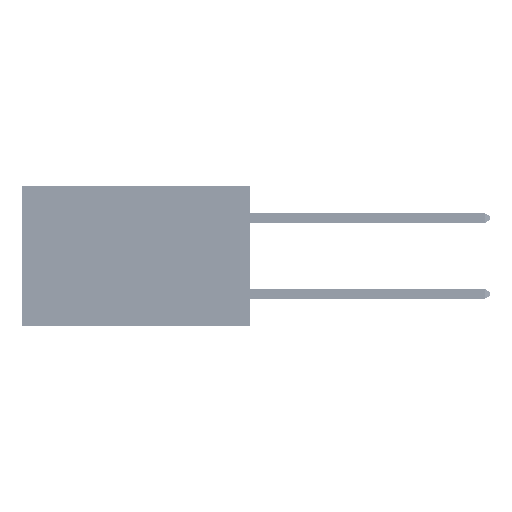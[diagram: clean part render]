
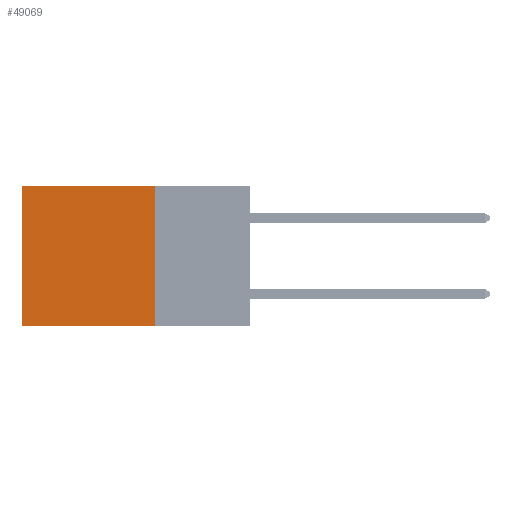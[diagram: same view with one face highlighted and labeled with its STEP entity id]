
A CAD part, left-side view. The second image highlights one B-rep face of the part: STEP entity #49069.
In plain terms, the highlighted planar face has unit normal (-1, 0, 0).
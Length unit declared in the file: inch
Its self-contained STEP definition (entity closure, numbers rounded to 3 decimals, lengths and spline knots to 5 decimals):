
#2378 = CARTESIAN_POINT ( 'NONE',  ( 0.2875, 0.6, 0. ) ) ;
#2854 = DIRECTION ( 'NONE',  ( 0., 1., 0. ) ) ;
#3376 = DIRECTION ( 'NONE',  ( 0., 0., -1. ) ) ;
#6018 = EDGE_LOOP ( 'NONE', ( #32790, #34989, #29587, #33026 ) ) ;
#6453 = LINE ( 'NONE', #21097, #10620 ) ;
#6478 = DIRECTION ( 'NONE',  ( 0., 0., -1. ) ) ;
#7643 = CARTESIAN_POINT ( 'NONE',  ( 0.2875, 0.25, 0. ) ) ;
#9830 = EDGE_CURVE ( 'NONE', #39778, #13255, #45789, .T. ) ;
#9989 = PLANE ( 'NONE',  #31469 ) ;
#10384 = VECTOR ( 'NONE', #3376, 39.37008 ) ;
#10620 = VECTOR ( 'NONE', #32876, 39.37008 ) ;
#13190 = VECTOR ( 'NONE', #18886, 39.37008 ) ;
#13255 = VERTEX_POINT ( 'NONE', #37118 ) ;
#15444 = EDGE_CURVE ( 'NONE', #17338, #19901, #24417, .T. ) ;
#17338 = VERTEX_POINT ( 'NONE', #34936 ) ;
#18886 = DIRECTION ( 'NONE',  ( 0., 1., 0. ) ) ;
#19901 = VERTEX_POINT ( 'NONE', #41632 ) ;
#21097 = CARTESIAN_POINT ( 'NONE',  ( 0.2875, 0.25, 0. ) ) ;
#23657 = EDGE_CURVE ( 'NONE', #39778, #17338, #6453, .T. ) ;
#24417 = LINE ( 'NONE', #32512, #26790 ) ;
#26790 = VECTOR ( 'NONE', #2854, 39.37008 ) ;
#29587 = ORIENTED_EDGE ( 'NONE', *, *, #23657, .F. ) ;
#31469 = AXIS2_PLACEMENT_3D ( 'NONE', #48266, #36786, #6478 ) ;
#31658 = FACE_OUTER_BOUND ( 'NONE', #6018, .T. ) ;
#31687 = LINE ( 'NONE', #2378, #10384 ) ;
#32512 = CARTESIAN_POINT ( 'NONE',  ( 0.2875, 0.25, -0.37 ) ) ;
#32790 = ORIENTED_EDGE ( 'NONE', *, *, #44866, .T. ) ;
#32876 = DIRECTION ( 'NONE',  ( 0., 0., -1. ) ) ;
#33026 = ORIENTED_EDGE ( 'NONE', *, *, #9830, .T. ) ;
#34936 = CARTESIAN_POINT ( 'NONE',  ( 0.2875, 0.25, -0.37 ) ) ;
#34989 = ORIENTED_EDGE ( 'NONE', *, *, #15444, .F. ) ;
#36786 = DIRECTION ( 'NONE',  ( 1., 0., 0. ) ) ;
#37118 = CARTESIAN_POINT ( 'NONE',  ( 0.2875, 0.6, 0. ) ) ;
#38499 = CARTESIAN_POINT ( 'NONE',  ( 0.2875, 0.25, 0. ) ) ;
#39778 = VERTEX_POINT ( 'NONE', #38499 ) ;
#41632 = CARTESIAN_POINT ( 'NONE',  ( 0.2875, 0.6, -0.37 ) ) ;
#44866 = EDGE_CURVE ( 'NONE', #13255, #19901, #31687, .T. ) ;
#45789 = LINE ( 'NONE', #7643, #13190 ) ;
#48266 = CARTESIAN_POINT ( 'NONE',  ( 0.2875, 0.25, 0. ) ) ;
#49069 = ADVANCED_FACE ( 'NONE', ( #31658 ), #9989, .F. ) ;
